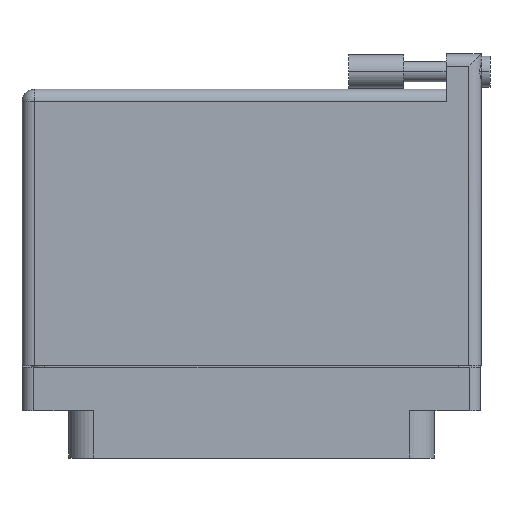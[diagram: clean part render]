
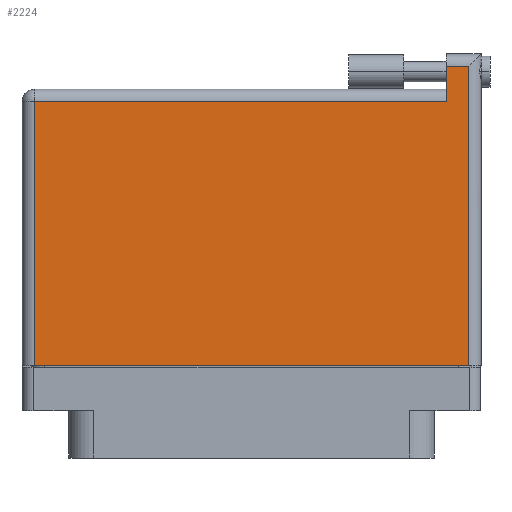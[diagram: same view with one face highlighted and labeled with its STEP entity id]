
A CAD part, front view. The second image highlights one B-rep face of the part: STEP entity #2224.
In plain terms, the highlighted face is planar.
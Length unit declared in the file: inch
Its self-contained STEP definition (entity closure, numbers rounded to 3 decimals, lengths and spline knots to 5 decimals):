
#62 = LINE ( 'NONE', #10104, #21282 ) ;
#722 = ORIENTED_EDGE ( 'NONE', *, *, #7540, .T. ) ;
#1256 = PLANE ( 'NONE',  #1350 ) ;
#1350 = AXIS2_PLACEMENT_3D ( 'NONE', #41321, #29215, #29563 ) ;
#1594 = CARTESIAN_POINT ( 'NONE',  ( 1.103, 1.596, 0.4495 ) ) ;
#2224 = ADVANCED_FACE ( 'NONE', ( #21950 ), #1256, .F. ) ;
#2343 = EDGE_CURVE ( 'NONE', #47612, #3260, #62, .T. ) ;
#2541 = DIRECTION ( 'NONE',  ( -1., 0., 0. ) ) ;
#2869 = VERTEX_POINT ( 'NONE', #22261 ) ;
#3260 = VERTEX_POINT ( 'NONE', #1594 ) ;
#4698 = VECTOR ( 'NONE', #50142, 39.37008 ) ;
#5156 = EDGE_CURVE ( 'NONE', #25231, #47612, #47985, .T. ) ;
#5890 = EDGE_CURVE ( 'NONE', #3260, #2869, #15930, .T. ) ;
#7540 = EDGE_CURVE ( 'NONE', #39338, #11305, #20759, .T. ) ;
#8493 = ORIENTED_EDGE ( 'NONE', *, *, #41983, .T. ) ;
#8548 = CARTESIAN_POINT ( 'NONE',  ( -1.23, -0.1, 0.4495 ) ) ;
#10076 = VECTOR ( 'NONE', #43655, 39.37008 ) ;
#10104 = CARTESIAN_POINT ( 'NONE',  ( -1.3, 1.596, 0.4495 ) ) ;
#11305 = VERTEX_POINT ( 'NONE', #8548 ) ;
#12503 = EDGE_LOOP ( 'NONE', ( #39467, #20445, #18718, #25997, #8493, #722 ) ) ;
#13062 = DIRECTION ( 'NONE',  ( 0., 1., 0. ) ) ;
#14200 = CARTESIAN_POINT ( 'NONE',  ( 1.23, 1.596, 0.4495 ) ) ;
#15307 = LINE ( 'NONE', #42154, #24704 ) ;
#15930 = LINE ( 'NONE', #41561, #4698 ) ;
#18020 = DIRECTION ( 'NONE',  ( -1., 0., 0. ) ) ;
#18718 = ORIENTED_EDGE ( 'NONE', *, *, #2343, .T. ) ;
#20445 = ORIENTED_EDGE ( 'NONE', *, *, #5156, .T. ) ;
#20759 = LINE ( 'NONE', #31553, #10076 ) ;
#21282 = VECTOR ( 'NONE', #18020, 39.37008 ) ;
#21950 = FACE_OUTER_BOUND ( 'NONE', #12503, .T. ) ;
#22261 = CARTESIAN_POINT ( 'NONE',  ( 1.103, 1.396, 0.4495 ) ) ;
#24704 = VECTOR ( 'NONE', #50385, 39.37008 ) ;
#25231 = VERTEX_POINT ( 'NONE', #40238 ) ;
#25997 = ORIENTED_EDGE ( 'NONE', *, *, #5890, .T. ) ;
#26158 = EDGE_CURVE ( 'NONE', #11305, #25231, #15307, .T. ) ;
#29215 = DIRECTION ( 'NONE',  ( 0., 0., -1. ) ) ;
#29563 = DIRECTION ( 'NONE',  ( -1., 0., 0. ) ) ;
#31095 = CARTESIAN_POINT ( 'NONE',  ( -1.23, 1.396, 0.4495 ) ) ;
#31553 = CARTESIAN_POINT ( 'NONE',  ( -1.23, -0.1, 0.4495 ) ) ;
#34691 = CARTESIAN_POINT ( 'NONE',  ( -1.3, 1.396, 0.4495 ) ) ;
#37434 = CARTESIAN_POINT ( 'NONE',  ( 1.23, 1.666, 0.4495 ) ) ;
#39338 = VERTEX_POINT ( 'NONE', #31095 ) ;
#39467 = ORIENTED_EDGE ( 'NONE', *, *, #26158, .T. ) ;
#40238 = CARTESIAN_POINT ( 'NONE',  ( 1.23, -0.1, 0.4495 ) ) ;
#40782 = LINE ( 'NONE', #34691, #43088 ) ;
#41321 = CARTESIAN_POINT ( 'NONE',  ( -1.3, 1.466, 0.4495 ) ) ;
#41561 = CARTESIAN_POINT ( 'NONE',  ( 1.103, 1.666, 0.4495 ) ) ;
#41983 = EDGE_CURVE ( 'NONE', #2869, #39338, #40782, .T. ) ;
#42154 = CARTESIAN_POINT ( 'NONE',  ( -1.3, -0.1, 0.4495 ) ) ;
#43088 = VECTOR ( 'NONE', #2541, 39.37008 ) ;
#43655 = DIRECTION ( 'NONE',  ( 0., -1., 0. ) ) ;
#47612 = VERTEX_POINT ( 'NONE', #14200 ) ;
#47985 = LINE ( 'NONE', #37434, #49860 ) ;
#49860 = VECTOR ( 'NONE', #13062, 39.37008 ) ;
#50142 = DIRECTION ( 'NONE',  ( 0., -1., 0. ) ) ;
#50385 = DIRECTION ( 'NONE',  ( 1., 0., 0. ) ) ;
